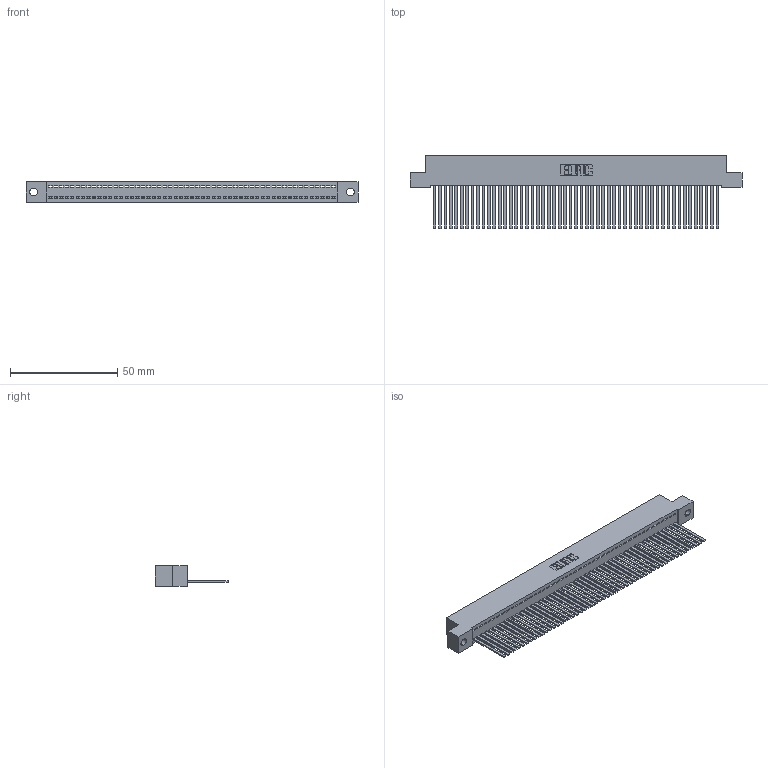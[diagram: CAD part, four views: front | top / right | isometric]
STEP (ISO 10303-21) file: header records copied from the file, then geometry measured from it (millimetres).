
FILE_DESCRIPTION (( 'STEP AP203' ), '1' );
FILE_NAME ('392-053-544-102.STEP', '2019-10-08T13:17:18', ( '' ), ( '' ), 'SwSTEP 2.0', 'SolidWorks 2016', '' );
FILE_SCHEMA (( 'CONFIG_CONTROL_DESIGN' ));
Length unit declared in the file: inch
Products named in the file (3): 345-292-001_345-293-144; 392-053-544-102; 342 Part_.128 Slot
Assembly tree (54 placements, depth 2):
  392-053-544-102
    342 Part_.128 Slot
    345-292-001_345-293-144  x53
Bounding box: 154.94 x 34.3 x 9.4 mm (x, y, z)
Volume: 14187.3 mm3; surface area: 22545.4 mm2
Topology: 54 solids, 54 shells, 2870 faces, 8685 edges, 5718 vertices
Faces by surface type: plane 2084, cylinder 786
Entity records: 30797 total; most frequent: CARTESIAN_POINT 5317, ORIENTED_EDGE 5306, DIRECTION 4459, EDGE_CURVE 2653, LINE 2529, VECTOR 2529, VERTEX_POINT 1766, AXIS2_PLACEMENT_3D 965
